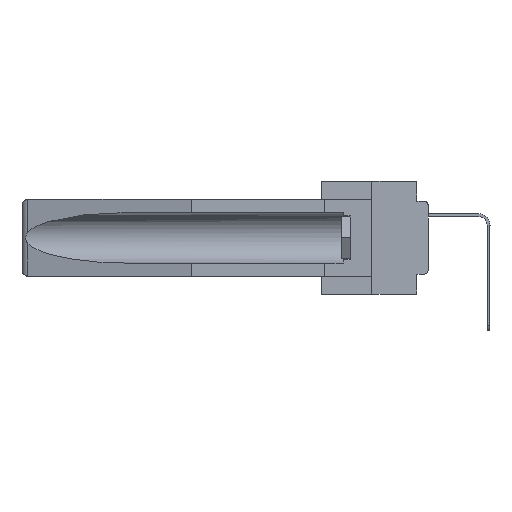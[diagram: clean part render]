
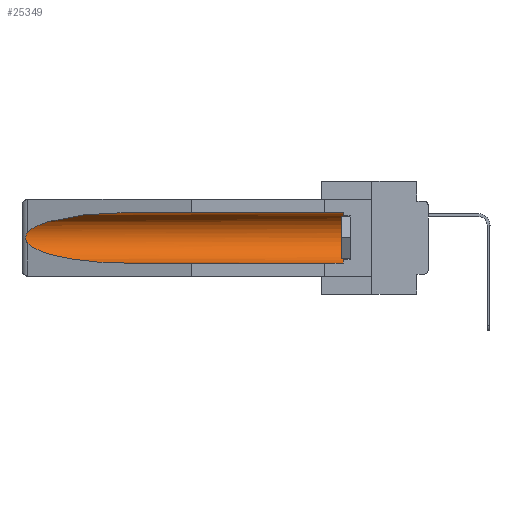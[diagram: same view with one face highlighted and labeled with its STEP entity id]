
A CAD part, left-side view. The second image highlights one B-rep face of the part: STEP entity #25349.
In plain terms, the highlighted cylindrical face has radius 2.857 mm (diameter 5.715 mm), a partial arc.
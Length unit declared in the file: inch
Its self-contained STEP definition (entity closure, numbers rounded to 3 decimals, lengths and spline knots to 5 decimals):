
#1459 = VERTEX_POINT ( 'NONE', #5469 ) ;
#1652 = CARTESIAN_POINT ( 'NONE',  ( 0.26537, 1.52718, -0.14972 ) ) ;
#2401 = CARTESIAN_POINT ( 'NONE',  ( 0.25451, 1.48313, -0.09465 ) ) ;
#2631 = DIRECTION ( 'NONE',  ( 0., 0., 1. ) ) ;
#3668 = ORIENTED_EDGE ( 'NONE', *, *, #14639, .T. ) ;
#3964 = EDGE_CURVE ( 'NONE', #1459, #36063, #28837, .T. ) ;
#4629 = CARTESIAN_POINT ( 'NONE',  ( 0.26654, 1.53092, -0.15636 ) ) ;
#5273 = EDGE_CURVE ( 'NONE', #12222, #6292, #10048, .T. ) ;
#5448 = EDGE_LOOP ( 'NONE', ( #32882, #19037, #24854, #22287, #30253, #3668 ) ) ;
#5469 = CARTESIAN_POINT ( 'NONE',  ( 0.26537, 1.52718, -0.19328 ) ) ;
#5677 = CARTESIAN_POINT ( 'NONE',  ( 0.155, 0.126, -0.059 ) ) ;
#6135 = VERTEX_POINT ( 'NONE', #32526 ) ;
#6292 = VERTEX_POINT ( 'NONE', #1652 ) ;
#6507 = EDGE_CURVE ( 'NONE', #6135, #36063, #33207, .T. ) ;
#7032 = CARTESIAN_POINT ( 'NONE',  ( 0.155, -0.30754, -0.059 ) ) ;
#8152 = CARTESIAN_POINT ( 'NONE',  ( 0.155, 0.126, -0.1715 ) ) ;
#8165 = CARTESIAN_POINT ( 'NONE',  ( 0.26537, 1.52718, -0.14972 ) ) ;
#8606 = VECTOR ( 'NONE', #33782, 39.37008 ) ;
#8666 = CARTESIAN_POINT ( 'NONE',  ( 0.21114, 1.30732, -0.059 ) ) ;
#9183 = CIRCLE ( 'NONE', #25962, 0.1125 ) ;
#9801 = EDGE_CURVE ( 'NONE', #6135, #24519, #9183, .T. ) ;
#10048 =( BOUNDED_CURVE ( )  B_SPLINE_CURVE ( 3, ( #16794, #8666, #2401, #8165 ),
 .UNSPECIFIED., .F., .F. ) 
 B_SPLINE_CURVE_WITH_KNOTS ( ( 4, 4 ),
 ( 4.71239, 6.08839 ),
 .UNSPECIFIED. ) 
 CURVE ( )  GEOMETRIC_REPRESENTATION_ITEM ( )  RATIONAL_B_SPLINE_CURVE ( ( 1., 0.848, 0.848, 1. ) ) 
 REPRESENTATION_ITEM ( '' )  );
#10392 = DIRECTION ( 'NONE',  ( 0., 1., 0. ) ) ;
#11283 = DIRECTION ( 'NONE',  ( 0., -1., 0. ) ) ;
#12222 = VERTEX_POINT ( 'NONE', #34056 ) ;
#13068 = CARTESIAN_POINT ( 'NONE',  ( 0.26655, 1.53094, -0.18657 ) ) ;
#13212 = AXIS2_PLACEMENT_3D ( 'NONE', #27488, #10392, #15766 ) ;
#14639 = EDGE_CURVE ( 'NONE', #24519, #12222, #18241, .T. ) ;
#15766 = DIRECTION ( 'NONE',  ( 0., 0., 1. ) ) ;
#15815 = CARTESIAN_POINT ( 'NONE',  ( 0.25451, 1.48313, -0.24835 ) ) ;
#15921 = CARTESIAN_POINT ( 'NONE',  ( 0.26537, 1.52718, -0.14972 ) ) ;
#16278 = CARTESIAN_POINT ( 'NONE',  ( 0.2675, 1.53308, -0.17534 ) ) ;
#16572 = EDGE_CURVE ( 'NONE', #6292, #1459, #25589, .T. ) ;
#16794 = CARTESIAN_POINT ( 'NONE',  ( 0.155, 1.07973, -0.059 ) ) ;
#17344 = VECTOR ( 'NONE', #21402, 39.37008 ) ;
#18241 = LINE ( 'NONE', #7032, #17344 ) ;
#18916 = CARTESIAN_POINT ( 'NONE',  ( 0.26597, 1.52961, -0.15275 ) ) ;
#19037 = ORIENTED_EDGE ( 'NONE', *, *, #16572, .T. ) ;
#21039 = CARTESIAN_POINT ( 'NONE',  ( 0.26537, 1.52718, -0.19328 ) ) ;
#21153 = CARTESIAN_POINT ( 'NONE',  ( 0.155, 1.07973, -0.284 ) ) ;
#21402 = DIRECTION ( 'NONE',  ( 0., 1., 0. ) ) ;
#22287 = ORIENTED_EDGE ( 'NONE', *, *, #6507, .F. ) ;
#23982 = FACE_OUTER_BOUND ( 'NONE', #5448, .T. ) ;
#24519 = VERTEX_POINT ( 'NONE', #5677 ) ;
#24854 = ORIENTED_EDGE ( 'NONE', *, *, #3964, .T. ) ;
#25349 = ADVANCED_FACE ( 'NONE', ( #23982 ), #35213, .F. ) ;
#25589 = B_SPLINE_CURVE_WITH_KNOTS ( 'NONE', 3,
 ( #15921, #18916, #4629, #33404, #30394, #16278, #36281, #13068, #30014, #33275 ),
 .UNSPECIFIED., .F., .F.,
 ( 4, 2, 2, 2, 4 ),
 ( 0., 0.00029, 0.00058, 0.00087, 0.00117 ),
 .UNSPECIFIED. ) ;
#25962 = AXIS2_PLACEMENT_3D ( 'NONE', #8152, #11283, #2631 ) ;
#27488 = CARTESIAN_POINT ( 'NONE',  ( 0.155, -0.30754, -0.1715 ) ) ;
#28837 =( BOUNDED_CURVE ( )  B_SPLINE_CURVE ( 3, ( #21039, #15815, #35806, #21153 ),
 .UNSPECIFIED., .F., .F. ) 
 B_SPLINE_CURVE_WITH_KNOTS ( ( 4, 4 ),
 ( 0.1948, 1.5708 ),
 .UNSPECIFIED. ) 
 CURVE ( )  GEOMETRIC_REPRESENTATION_ITEM ( )  RATIONAL_B_SPLINE_CURVE ( ( 1., 0.848, 0.848, 1. ) ) 
 REPRESENTATION_ITEM ( '' )  );
#30014 = CARTESIAN_POINT ( 'NONE',  ( 0.26597, 1.5296, -0.19026 ) ) ;
#30253 = ORIENTED_EDGE ( 'NONE', *, *, #9801, .T. ) ;
#30394 = CARTESIAN_POINT ( 'NONE',  ( 0.2675, 1.53308, -0.16763 ) ) ;
#32526 = CARTESIAN_POINT ( 'NONE',  ( 0.155, 0.126, -0.284 ) ) ;
#32882 = ORIENTED_EDGE ( 'NONE', *, *, #5273, .T. ) ;
#33207 = LINE ( 'NONE', #33910, #8606 ) ;
#33275 = CARTESIAN_POINT ( 'NONE',  ( 0.26537, 1.52718, -0.19328 ) ) ;
#33404 = CARTESIAN_POINT ( 'NONE',  ( 0.2673, 1.5327, -0.16383 ) ) ;
#33782 = DIRECTION ( 'NONE',  ( 0., 1., 0. ) ) ;
#33910 = CARTESIAN_POINT ( 'NONE',  ( 0.155, -0.30754, -0.284 ) ) ;
#34056 = CARTESIAN_POINT ( 'NONE',  ( 0.155, 1.07973, -0.059 ) ) ;
#34912 = CARTESIAN_POINT ( 'NONE',  ( 0.155, 1.07973, -0.284 ) ) ;
#35213 = CYLINDRICAL_SURFACE ( 'NONE', #13212, 0.1125 ) ;
#35806 = CARTESIAN_POINT ( 'NONE',  ( 0.21114, 1.30732, -0.284 ) ) ;
#36063 = VERTEX_POINT ( 'NONE', #34912 ) ;
#36281 = CARTESIAN_POINT ( 'NONE',  ( 0.2673, 1.53269, -0.17917 ) ) ;
